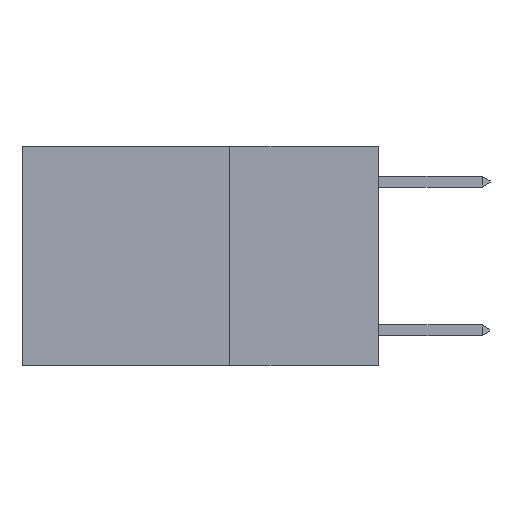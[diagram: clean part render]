
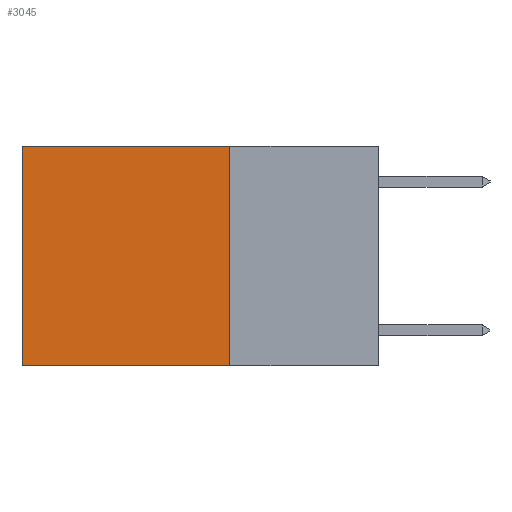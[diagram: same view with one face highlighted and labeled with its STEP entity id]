
A CAD part, left-side view. The second image highlights one B-rep face of the part: STEP entity #3045.
In plain terms, the highlighted planar face has unit normal (-1, 0, 0).
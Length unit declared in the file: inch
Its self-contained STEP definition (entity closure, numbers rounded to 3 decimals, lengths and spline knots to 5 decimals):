
#203 = DIRECTION ( 'NONE',  ( 0., 0., -1. ) ) ;
#439 = EDGE_CURVE ( 'NONE', #2853, #7646, #4120, .T. ) ;
#471 = EDGE_CURVE ( 'NONE', #2853, #6412, #2764, .T. ) ;
#527 = CARTESIAN_POINT ( 'NONE',  ( 0.2625, 0.25, 0. ) ) ;
#1094 = ORIENTED_EDGE ( 'NONE', *, *, #2808, .T. ) ;
#1143 = ORIENTED_EDGE ( 'NONE', *, *, #6138, .F. ) ;
#1472 = CARTESIAN_POINT ( 'NONE',  ( 0.2625, 0.6, 0. ) ) ;
#1513 = EDGE_LOOP ( 'NONE', ( #1094, #1143, #2279, #1603 ) ) ;
#1603 = ORIENTED_EDGE ( 'NONE', *, *, #471, .T. ) ;
#2279 = ORIENTED_EDGE ( 'NONE', *, *, #439, .F. ) ;
#2764 = LINE ( 'NONE', #527, #4311 ) ;
#2808 = EDGE_CURVE ( 'NONE', #6412, #4727, #4609, .T. ) ;
#2819 = CARTESIAN_POINT ( 'NONE',  ( 0.2625, 0.25, 0. ) ) ;
#2827 = DIRECTION ( 'NONE',  ( 0., 1., 0. ) ) ;
#2853 = VERTEX_POINT ( 'NONE', #7591 ) ;
#2854 = CARTESIAN_POINT ( 'NONE',  ( 0.2625, 0.25, -0.37 ) ) ;
#2919 = FACE_OUTER_BOUND ( 'NONE', #1513, .T. ) ;
#3045 = ADVANCED_FACE ( 'NONE', ( #2919 ), #8298, .F. ) ;
#4120 = LINE ( 'NONE', #2819, #6639 ) ;
#4311 = VECTOR ( 'NONE', #6478, 39.37008 ) ;
#4609 = LINE ( 'NONE', #8234, #4709 ) ;
#4709 = VECTOR ( 'NONE', #8215, 39.37008 ) ;
#4727 = VERTEX_POINT ( 'NONE', #7530 ) ;
#6138 = EDGE_CURVE ( 'NONE', #7646, #4727, #7905, .T. ) ;
#6412 = VERTEX_POINT ( 'NONE', #1472 ) ;
#6478 = DIRECTION ( 'NONE',  ( 0., 1., 0. ) ) ;
#6639 = VECTOR ( 'NONE', #203, 39.37008 ) ;
#7419 = CARTESIAN_POINT ( 'NONE',  ( 0.2625, 0.25, -0.37 ) ) ;
#7530 = CARTESIAN_POINT ( 'NONE',  ( 0.2625, 0.6, -0.37 ) ) ;
#7591 = CARTESIAN_POINT ( 'NONE',  ( 0.2625, 0.25, 0. ) ) ;
#7646 = VERTEX_POINT ( 'NONE', #7419 ) ;
#7807 = VECTOR ( 'NONE', #2827, 39.37008 ) ;
#7905 = LINE ( 'NONE', #2854, #7807 ) ;
#8178 = AXIS2_PLACEMENT_3D ( 'NONE', #8266, #8224, #8204 ) ;
#8204 = DIRECTION ( 'NONE',  ( 0., 0., -1. ) ) ;
#8215 = DIRECTION ( 'NONE',  ( 0., 0., -1. ) ) ;
#8224 = DIRECTION ( 'NONE',  ( 1., 0., 0. ) ) ;
#8234 = CARTESIAN_POINT ( 'NONE',  ( 0.2625, 0.6, 0. ) ) ;
#8266 = CARTESIAN_POINT ( 'NONE',  ( 0.2625, 0.25, 0. ) ) ;
#8298 = PLANE ( 'NONE',  #8178 ) ;
